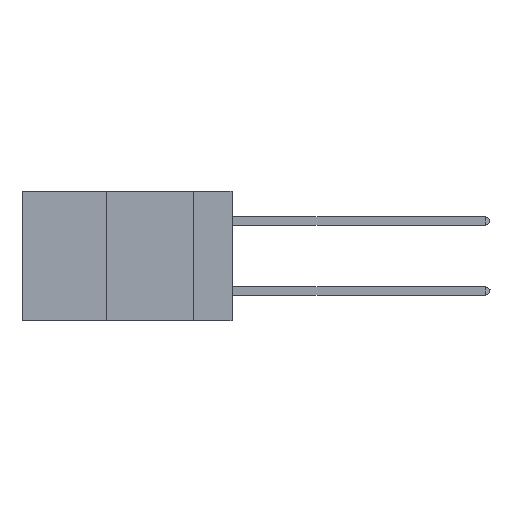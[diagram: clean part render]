
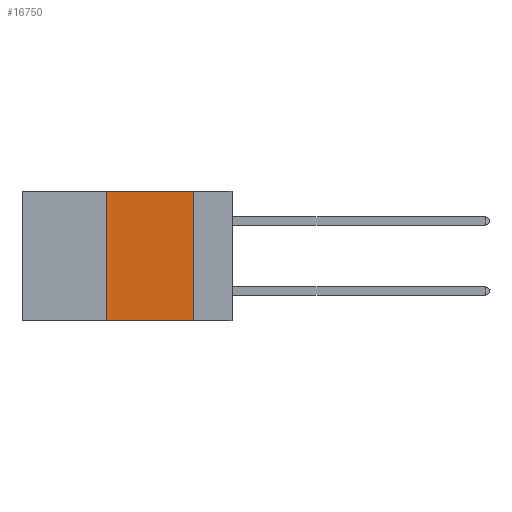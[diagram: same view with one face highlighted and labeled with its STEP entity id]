
A CAD part, left-side view. The second image highlights one B-rep face of the part: STEP entity #16750.
In plain terms, the highlighted planar face has unit normal (-1, 0, 0).
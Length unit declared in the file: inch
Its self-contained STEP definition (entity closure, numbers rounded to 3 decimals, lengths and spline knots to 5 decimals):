
#498 = ORIENTED_EDGE ( 'NONE', *, *, #18667, .T. ) ;
#1882 = CARTESIAN_POINT ( 'NONE',  ( 0., 0.11, 0. ) ) ;
#2165 = PLANE ( 'NONE',  #3274 ) ;
#3274 = AXIS2_PLACEMENT_3D ( 'NONE', #5553, #12778, #10936 ) ;
#4023 = ORIENTED_EDGE ( 'NONE', *, *, #12215, .F. ) ;
#5006 = VECTOR ( 'NONE', #16257, 39.37008 ) ;
#5102 = ORIENTED_EDGE ( 'NONE', *, *, #8298, .F. ) ;
#5553 = CARTESIAN_POINT ( 'NONE',  ( 0., 0.6, 0. ) ) ;
#6233 = EDGE_CURVE ( 'NONE', #7955, #8364, #20778, .T. ) ;
#6889 = LINE ( 'NONE', #1882, #15929 ) ;
#7342 = CARTESIAN_POINT ( 'NONE',  ( 0., 0.36, 0. ) ) ;
#7955 = VERTEX_POINT ( 'NONE', #7342 ) ;
#8298 = EDGE_CURVE ( 'NONE', #8364, #19653, #6889, .T. ) ;
#8364 = VERTEX_POINT ( 'NONE', #18822 ) ;
#8751 = LINE ( 'NONE', #20165, #13970 ) ;
#9706 = LINE ( 'NONE', #16476, #5006 ) ;
#10936 = DIRECTION ( 'NONE',  ( 0., 0., -1. ) ) ;
#11746 = ORIENTED_EDGE ( 'NONE', *, *, #6233, .F. ) ;
#11910 = VECTOR ( 'NONE', #19224, 39.37008 ) ;
#12215 = EDGE_CURVE ( 'NONE', #13687, #7955, #8751, .T. ) ;
#12778 = DIRECTION ( 'NONE',  ( 1., 0., 0. ) ) ;
#13687 = VERTEX_POINT ( 'NONE', #21953 ) ;
#13970 = VECTOR ( 'NONE', #16899, 39.37008 ) ;
#15929 = VECTOR ( 'NONE', #19113, 39.37008 ) ;
#16257 = DIRECTION ( 'NONE',  ( 0., -1., 0. ) ) ;
#16476 = CARTESIAN_POINT ( 'NONE',  ( 0., 0.6, -0.37 ) ) ;
#16750 = ADVANCED_FACE ( 'NONE', ( #19448 ), #2165, .F. ) ;
#16899 = DIRECTION ( 'NONE',  ( 0., 0., 1. ) ) ;
#18667 = EDGE_CURVE ( 'NONE', #13687, #19653, #9706, .T. ) ;
#18822 = CARTESIAN_POINT ( 'NONE',  ( 0., 0.11, 0. ) ) ;
#19113 = DIRECTION ( 'NONE',  ( 0., 0., -1. ) ) ;
#19152 = CARTESIAN_POINT ( 'NONE',  ( 0., 0.6, 0. ) ) ;
#19224 = DIRECTION ( 'NONE',  ( 0., -1., 0. ) ) ;
#19448 = FACE_OUTER_BOUND ( 'NONE', #19646, .T. ) ;
#19646 = EDGE_LOOP ( 'NONE', ( #5102, #11746, #4023, #498 ) ) ;
#19653 = VERTEX_POINT ( 'NONE', #20118 ) ;
#20118 = CARTESIAN_POINT ( 'NONE',  ( 0., 0.11, -0.37 ) ) ;
#20165 = CARTESIAN_POINT ( 'NONE',  ( 0., 0.36, 0. ) ) ;
#20778 = LINE ( 'NONE', #19152, #11910 ) ;
#21953 = CARTESIAN_POINT ( 'NONE',  ( 0., 0.36, -0.37 ) ) ;
